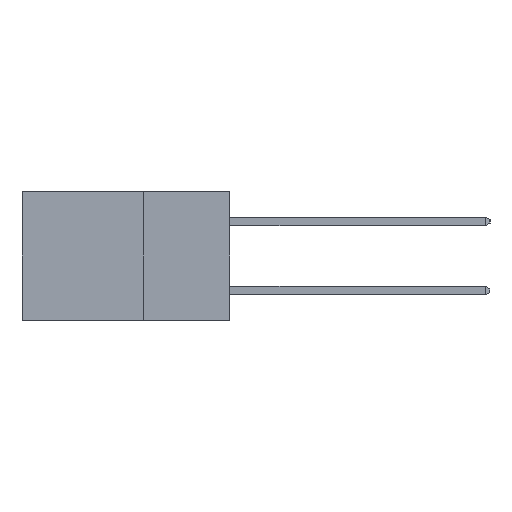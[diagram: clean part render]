
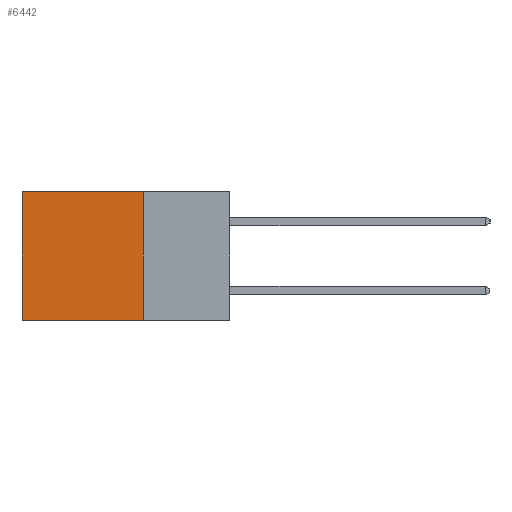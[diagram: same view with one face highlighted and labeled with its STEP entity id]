
A CAD part, left-side view. The second image highlights one B-rep face of the part: STEP entity #6442.
In plain terms, the highlighted planar face has unit normal (-1, 0, 0).
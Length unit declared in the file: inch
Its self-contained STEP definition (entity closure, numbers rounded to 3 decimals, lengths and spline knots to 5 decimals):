
#81 = LINE ( 'NONE', #13027, #10894 ) ;
#437 = DIRECTION ( 'NONE',  ( 1., 0., 0. ) ) ;
#2476 = EDGE_CURVE ( 'NONE', #7772, #3573, #9022, .T. ) ;
#2720 = CARTESIAN_POINT ( 'NONE',  ( 0.298, 0.25, 0. ) ) ;
#2993 = ORIENTED_EDGE ( 'NONE', *, *, #5805, .F. ) ;
#3573 = VERTEX_POINT ( 'NONE', #4926 ) ;
#3612 = CARTESIAN_POINT ( 'NONE',  ( 0.298, 0.25, -0.37 ) ) ;
#3647 = CARTESIAN_POINT ( 'NONE',  ( 0.298, 0.6, 0. ) ) ;
#3679 = DIRECTION ( 'NONE',  ( 0., 1., 0. ) ) ;
#3917 = VECTOR ( 'NONE', #8804, 39.37008 ) ;
#4026 = FACE_OUTER_BOUND ( 'NONE', #12219, .T. ) ;
#4611 = CARTESIAN_POINT ( 'NONE',  ( 0.298, 0.25, 0. ) ) ;
#4698 = VERTEX_POINT ( 'NONE', #2720 ) ;
#4926 = CARTESIAN_POINT ( 'NONE',  ( 0.298, 0.6, -0.37 ) ) ;
#5805 = EDGE_CURVE ( 'NONE', #4698, #7773, #81, .T. ) ;
#6221 = VECTOR ( 'NONE', #7468, 39.37008 ) ;
#6442 = ADVANCED_FACE ( 'NONE', ( #4026 ), #6691, .F. ) ;
#6658 = LINE ( 'NONE', #3612, #3917 ) ;
#6691 = PLANE ( 'NONE',  #11222 ) ;
#6955 = ORIENTED_EDGE ( 'NONE', *, *, #10623, .F. ) ;
#7143 = ORIENTED_EDGE ( 'NONE', *, *, #10078, .T. ) ;
#7341 = LINE ( 'NONE', #10983, #10128 ) ;
#7468 = DIRECTION ( 'NONE',  ( 0., 0., -1. ) ) ;
#7758 = DIRECTION ( 'NONE',  ( 0., 0., -1. ) ) ;
#7772 = VERTEX_POINT ( 'NONE', #13074 ) ;
#7773 = VERTEX_POINT ( 'NONE', #11041 ) ;
#8804 = DIRECTION ( 'NONE',  ( 0., 1., 0. ) ) ;
#9022 = LINE ( 'NONE', #3647, #6221 ) ;
#9931 = DIRECTION ( 'NONE',  ( 0., 0., -1. ) ) ;
#10054 = ORIENTED_EDGE ( 'NONE', *, *, #2476, .T. ) ;
#10078 = EDGE_CURVE ( 'NONE', #4698, #7772, #7341, .T. ) ;
#10128 = VECTOR ( 'NONE', #3679, 39.37008 ) ;
#10623 = EDGE_CURVE ( 'NONE', #7773, #3573, #6658, .T. ) ;
#10894 = VECTOR ( 'NONE', #9931, 39.37008 ) ;
#10983 = CARTESIAN_POINT ( 'NONE',  ( 0.298, 0.25, 0. ) ) ;
#11041 = CARTESIAN_POINT ( 'NONE',  ( 0.298, 0.25, -0.37 ) ) ;
#11222 = AXIS2_PLACEMENT_3D ( 'NONE', #4611, #437, #7758 ) ;
#12219 = EDGE_LOOP ( 'NONE', ( #10054, #6955, #2993, #7143 ) ) ;
#13027 = CARTESIAN_POINT ( 'NONE',  ( 0.298, 0.25, 0. ) ) ;
#13074 = CARTESIAN_POINT ( 'NONE',  ( 0.298, 0.6, 0. ) ) ;
